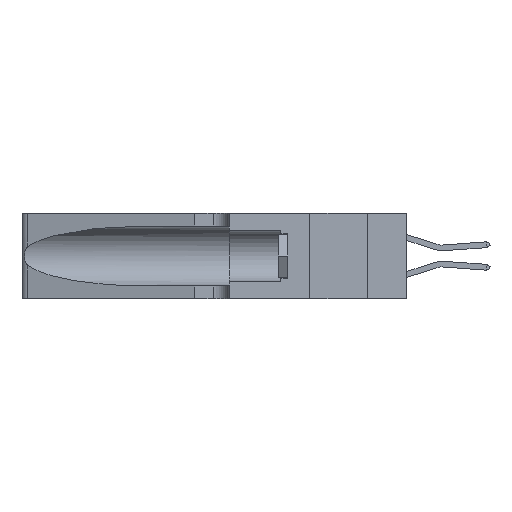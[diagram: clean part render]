
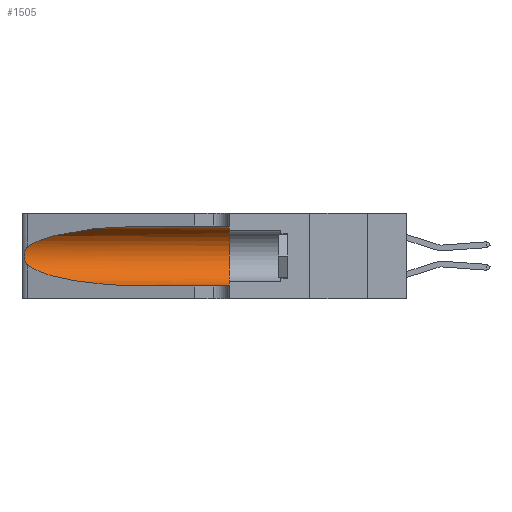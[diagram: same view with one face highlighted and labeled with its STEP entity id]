
A CAD part, left-side view. The second image highlights one B-rep face of the part: STEP entity #1505.
In plain terms, the highlighted cylindrical face has radius 3.308 mm (diameter 6.617 mm), a partial arc.
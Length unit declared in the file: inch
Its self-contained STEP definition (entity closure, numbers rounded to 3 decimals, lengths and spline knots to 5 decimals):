
#720 = CARTESIAN_POINT ( 'NONE',  ( 0.25487, 1.22718, 0.14631 ) ) ;
#1148 = CARTESIAN_POINT ( 'NONE',  ( 0.1305, 0.35, 0.05475 ) ) ;
#1361 = LINE ( 'NONE', #18300, #24369 ) ;
#1505 = ADVANCED_FACE ( 'NONE', ( #11424 ), #22508, .F. ) ;
#1977 = CARTESIAN_POINT ( 'NONE',  ( 0.26075, 1.23896, 0.178 ) ) ;
#1987 = LINE ( 'NONE', #27877, #19130 ) ;
#3120 = CARTESIAN_POINT ( 'NONE',  ( 0.18966, 0.96281, 0.05475 ) ) ;
#3378 = CARTESIAN_POINT ( 'NONE',  ( 0.18966, 0.96281, 0.31525 ) ) ;
#3788 = VERTEX_POINT ( 'NONE', #18991 ) ;
#3887 = ORIENTED_EDGE ( 'NONE', *, *, #20243, .T. ) ;
#4297 = CARTESIAN_POINT ( 'NONE',  ( 0.25856, 1.23593, 0.16098 ) ) ;
#4602 = CARTESIAN_POINT ( 'NONE',  ( 0.1305, 1.61858, 0.185 ) ) ;
#4926 = VERTEX_POINT ( 'NONE', #23755 ) ;
#5621 = AXIS2_PLACEMENT_3D ( 'NONE', #4602, #24494, #17918 ) ;
#5825 = CIRCLE ( 'NONE', #8067, 0.13025 ) ;
#6552 = CARTESIAN_POINT ( 'NONE',  ( 0.25639, 1.23186, 0.15144 ) ) ;
#6844 = VERTEX_POINT ( 'NONE', #1148 ) ;
#6974 = ORIENTED_EDGE ( 'NONE', *, *, #10974, .F. ) ;
#7927 = DIRECTION ( 'NONE',  ( 0., -1., 0. ) ) ;
#8067 = AXIS2_PLACEMENT_3D ( 'NONE', #10039, #25563, #12296 ) ;
#8784 = CARTESIAN_POINT ( 'NONE',  ( 0.25487, 1.22718, 0.14631 ) ) ;
#9460 = DIRECTION ( 'NONE',  ( 0., -1., 0. ) ) ;
#10039 = CARTESIAN_POINT ( 'NONE',  ( 0.1305, 0.35, 0.185 ) ) ;
#10109 = CARTESIAN_POINT ( 'NONE',  ( 0.2373, 1.15595, 0.28018 ) ) ;
#10907 = CARTESIAN_POINT ( 'NONE',  ( 0.25639, 1.23184, 0.21858 ) ) ;
#10974 = EDGE_CURVE ( 'NONE', #25172, #4926, #1361, .T. ) ;
#11424 = FACE_OUTER_BOUND ( 'NONE', #14635, .T. ) ;
#12296 = DIRECTION ( 'NONE',  ( 0., 0., 1. ) ) ;
#13161 = CARTESIAN_POINT ( 'NONE',  ( 0.25854, 1.2359, 0.20912 ) ) ;
#14250 = CARTESIAN_POINT ( 'NONE',  ( 0.2373, 1.15595, 0.08982 ) ) ;
#14635 = EDGE_LOOP ( 'NONE', ( #21778, #23346, #16211, #3887, #23532, #6974 ) ) ;
#15293 = CARTESIAN_POINT ( 'NONE',  ( 0.25487, 1.22718, 0.22369 ) ) ;
#15397 = CARTESIAN_POINT ( 'NONE',  ( 0.26075, 1.23896, 0.19203 ) ) ;
#15436 = EDGE_CURVE ( 'NONE', #4926, #6844, #5825, .T. ) ;
#15891 = CARTESIAN_POINT ( 'NONE',  ( 0.1305, 0.72297, 0.05475 ) ) ;
#16198 = B_SPLINE_CURVE_WITH_KNOTS ( 'NONE', 3,
 ( #15293, #28539, #10907, #26415, #13161, #28633, #15397, #1977, #17622, #4297, #19846, #6552, #22056, #8784 ),
 .UNSPECIFIED., .F., .F.,
 ( 4, 2, 2, 2, 2, 2, 4 ),
 ( 0., 0.00027, 0.00053, 0.00107, 0.0016, 0.00187, 0.00214 ),
 .UNSPECIFIED. ) ;
#16211 = ORIENTED_EDGE ( 'NONE', *, *, #19215, .T. ) ;
#17622 = CARTESIAN_POINT ( 'NONE',  ( 0.26017, 1.23833, 0.17102 ) ) ;
#17918 = DIRECTION ( 'NONE',  ( 0., 0., -1. ) ) ;
#18300 = CARTESIAN_POINT ( 'NONE',  ( 0.1305, 1.61858, 0.31525 ) ) ;
#18712 = CARTESIAN_POINT ( 'NONE',  ( 0.1305, 0.72297, 0.05475 ) ) ;
#18872 = CARTESIAN_POINT ( 'NONE',  ( 0.1305, 0.72297, 0.31525 ) ) ;
#18991 = CARTESIAN_POINT ( 'NONE',  ( 0.25487, 1.22718, 0.14631 ) ) ;
#19130 = VECTOR ( 'NONE', #7927, 39.37008 ) ;
#19215 = EDGE_CURVE ( 'NONE', #3788, #19958, #23461, .T. ) ;
#19846 = CARTESIAN_POINT ( 'NONE',  ( 0.25789, 1.23486, 0.15765 ) ) ;
#19958 = VERTEX_POINT ( 'NONE', #15891 ) ;
#20243 = EDGE_CURVE ( 'NONE', #19958, #6844, #1987, .T. ) ;
#21231 = CARTESIAN_POINT ( 'NONE',  ( 0.1305, 0.72297, 0.31525 ) ) ;
#21340 =( BOUNDED_CURVE ( )  B_SPLINE_CURVE ( 3, ( #18872, #3378, #10109, #25624 ),
 .UNSPECIFIED., .F., .F. ) 
 B_SPLINE_CURVE_WITH_KNOTS ( ( 4, 4 ),
 ( 1.5708, 2.84003 ),
 .UNSPECIFIED. ) 
 CURVE ( )  GEOMETRIC_REPRESENTATION_ITEM ( )  RATIONAL_B_SPLINE_CURVE ( ( 1., 0.87, 0.87, 1. ) ) 
 REPRESENTATION_ITEM ( '' )  );
#21778 = ORIENTED_EDGE ( 'NONE', *, *, #26518, .T. ) ;
#22056 = CARTESIAN_POINT ( 'NONE',  ( 0.25555, 1.22993, 0.14849 ) ) ;
#22508 = CYLINDRICAL_SURFACE ( 'NONE', #5621, 0.13025 ) ;
#23346 = ORIENTED_EDGE ( 'NONE', *, *, #27995, .T. ) ;
#23461 =( BOUNDED_CURVE ( )  B_SPLINE_CURVE ( 3, ( #720, #14250, #3120, #18712 ),
 .UNSPECIFIED., .F., .F. ) 
 B_SPLINE_CURVE_WITH_KNOTS ( ( 4, 4 ),
 ( 3.44316, 4.71239 ),
 .UNSPECIFIED. ) 
 CURVE ( )  GEOMETRIC_REPRESENTATION_ITEM ( )  RATIONAL_B_SPLINE_CURVE ( ( 1., 0.87, 0.87, 1. ) ) 
 REPRESENTATION_ITEM ( '' )  );
#23532 = ORIENTED_EDGE ( 'NONE', *, *, #15436, .F. ) ;
#23755 = CARTESIAN_POINT ( 'NONE',  ( 0.1305, 0.35, 0.31525 ) ) ;
#23921 = VERTEX_POINT ( 'NONE', #28059 ) ;
#24369 = VECTOR ( 'NONE', #9460, 39.37008 ) ;
#24494 = DIRECTION ( 'NONE',  ( 0., -1., 0. ) ) ;
#25172 = VERTEX_POINT ( 'NONE', #21231 ) ;
#25563 = DIRECTION ( 'NONE',  ( 0., 1., 0. ) ) ;
#25624 = CARTESIAN_POINT ( 'NONE',  ( 0.25487, 1.22718, 0.22369 ) ) ;
#26415 = CARTESIAN_POINT ( 'NONE',  ( 0.25787, 1.23484, 0.2124 ) ) ;
#26518 = EDGE_CURVE ( 'NONE', #25172, #23921, #21340, .T. ) ;
#27877 = CARTESIAN_POINT ( 'NONE',  ( 0.1305, 1.61858, 0.05475 ) ) ;
#27995 = EDGE_CURVE ( 'NONE', #23921, #3788, #16198, .T. ) ;
#28059 = CARTESIAN_POINT ( 'NONE',  ( 0.25487, 1.22718, 0.22369 ) ) ;
#28539 = CARTESIAN_POINT ( 'NONE',  ( 0.25555, 1.22994, 0.2215 ) ) ;
#28633 = CARTESIAN_POINT ( 'NONE',  ( 0.26018, 1.23835, 0.19895 ) ) ;
